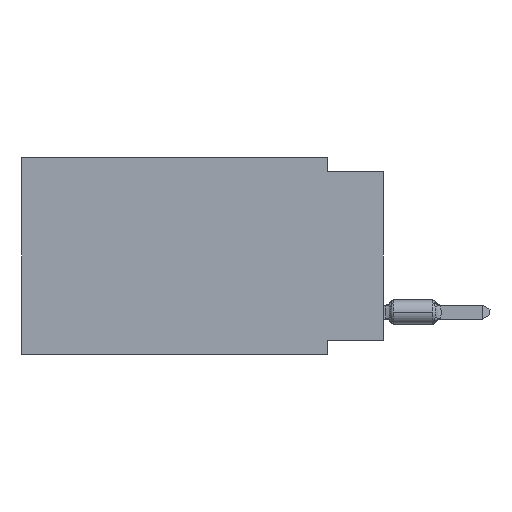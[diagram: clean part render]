
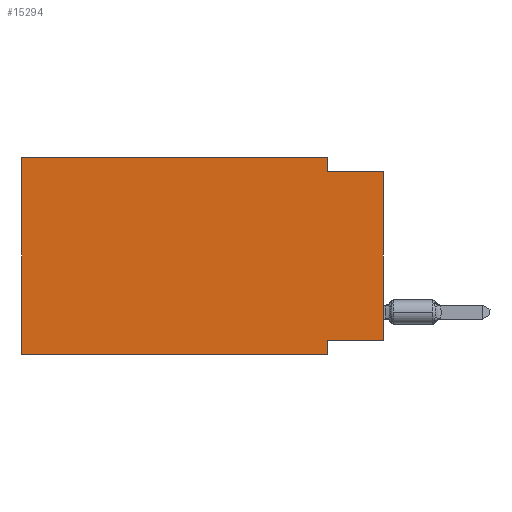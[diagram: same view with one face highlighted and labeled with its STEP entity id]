
A CAD part, left-side view. The second image highlights one B-rep face of the part: STEP entity #15294.
In plain terms, the highlighted planar face has unit normal (-1, 0, 0).
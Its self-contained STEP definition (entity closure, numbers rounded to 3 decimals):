
#206 = VERTEX_POINT ( 'NONE', #7368 ) ;
#236 = CARTESIAN_POINT ( 'NONE',  ( 0., 16.383, 0. ) ) ;
#322 = CARTESIAN_POINT ( 'NONE',  ( 0., 2.54, -8.89 ) ) ;
#358 = VECTOR ( 'NONE', #21157, 1000. ) ;
#823 = VERTEX_POINT ( 'NONE', #1305 ) ;
#853 = VERTEX_POINT ( 'NONE', #322 ) ;
#1194 = LINE ( 'NONE', #21129, #14023 ) ;
#1305 = CARTESIAN_POINT ( 'NONE',  ( 0., 0., -0.635 ) ) ;
#1414 = DIRECTION ( 'NONE',  ( 0., 1., 0. ) ) ;
#1846 = CARTESIAN_POINT ( 'NONE',  ( 0., 0., -0.635 ) ) ;
#2384 = VECTOR ( 'NONE', #6241, 1000. ) ;
#2783 = ORIENTED_EDGE ( 'NONE', *, *, #10857, .T. ) ;
#2955 = CARTESIAN_POINT ( 'NONE',  ( 0., 0., -8.255 ) ) ;
#3058 = ORIENTED_EDGE ( 'NONE', *, *, #7679, .F. ) ;
#3136 = LINE ( 'NONE', #18038, #358 ) ;
#3513 = VECTOR ( 'NONE', #8392, 1000. ) ;
#3583 = ORIENTED_EDGE ( 'NONE', *, *, #16313, .F. ) ;
#3991 = VECTOR ( 'NONE', #20183, 1000. ) ;
#4139 = LINE ( 'NONE', #14010, #7663 ) ;
#4697 = CARTESIAN_POINT ( 'NONE',  ( 0., 16.383, -8.89 ) ) ;
#5078 = EDGE_CURVE ( 'NONE', #13953, #853, #3136, .T. ) ;
#5245 = VERTEX_POINT ( 'NONE', #236 ) ;
#6067 = AXIS2_PLACEMENT_3D ( 'NONE', #10960, #11172, #17395 ) ;
#6167 = VERTEX_POINT ( 'NONE', #20225 ) ;
#6241 = DIRECTION ( 'NONE',  ( 0., 0., 1. ) ) ;
#7368 = CARTESIAN_POINT ( 'NONE',  ( 0., 2.54, -0.635 ) ) ;
#7663 = VECTOR ( 'NONE', #17224, 1000. ) ;
#7679 = EDGE_CURVE ( 'NONE', #206, #823, #18147, .T. ) ;
#7737 = DIRECTION ( 'NONE',  ( 0., -1., 0. ) ) ;
#8152 = EDGE_CURVE ( 'NONE', #19121, #13953, #19838, .T. ) ;
#8179 = CARTESIAN_POINT ( 'NONE',  ( 0., 2.54, 0. ) ) ;
#8392 = DIRECTION ( 'NONE',  ( 0., -1., 0. ) ) ;
#8438 = EDGE_LOOP ( 'NONE', ( #2783, #3058, #14047, #13711, #3583, #16849, #16554, #11705 ) ) ;
#8721 = LINE ( 'NONE', #13652, #3991 ) ;
#9462 = CARTESIAN_POINT ( 'NONE',  ( 0., 0., 0. ) ) ;
#9680 = FACE_OUTER_BOUND ( 'NONE', #8438, .T. ) ;
#9781 = CARTESIAN_POINT ( 'NONE',  ( 0., 0., -8.255 ) ) ;
#10857 = EDGE_CURVE ( 'NONE', #19121, #823, #21034, .T. ) ;
#10960 = CARTESIAN_POINT ( 'NONE',  ( 0., 16.383, 0. ) ) ;
#11172 = DIRECTION ( 'NONE',  ( 1., 0., 0. ) ) ;
#11208 = EDGE_CURVE ( 'NONE', #6167, #853, #19391, .T. ) ;
#11239 = DIRECTION ( 'NONE',  ( 0., -1., 0. ) ) ;
#11705 = ORIENTED_EDGE ( 'NONE', *, *, #8152, .F. ) ;
#12894 = PLANE ( 'NONE',  #6067 ) ;
#13652 = CARTESIAN_POINT ( 'NONE',  ( 0., 16.383, 0. ) ) ;
#13711 = ORIENTED_EDGE ( 'NONE', *, *, #14852, .F. ) ;
#13953 = VERTEX_POINT ( 'NONE', #14702 ) ;
#14010 = CARTESIAN_POINT ( 'NONE',  ( 0., 2.54, 0. ) ) ;
#14023 = VECTOR ( 'NONE', #7737, 1000. ) ;
#14047 = ORIENTED_EDGE ( 'NONE', *, *, #20196, .F. ) ;
#14702 = CARTESIAN_POINT ( 'NONE',  ( 0., 2.54, -8.255 ) ) ;
#14852 = EDGE_CURVE ( 'NONE', #5245, #17685, #1194, .T. ) ;
#15294 = ADVANCED_FACE ( 'NONE', ( #9680 ), #12894, .F. ) ;
#16313 = EDGE_CURVE ( 'NONE', #6167, #5245, #8721, .T. ) ;
#16554 = ORIENTED_EDGE ( 'NONE', *, *, #5078, .F. ) ;
#16849 = ORIENTED_EDGE ( 'NONE', *, *, #11208, .T. ) ;
#17222 = VECTOR ( 'NONE', #1414, 1000. ) ;
#17224 = DIRECTION ( 'NONE',  ( 0., 0., -1. ) ) ;
#17395 = DIRECTION ( 'NONE',  ( 0., 0., -1. ) ) ;
#17413 = VECTOR ( 'NONE', #11239, 1000. ) ;
#17685 = VERTEX_POINT ( 'NONE', #8179 ) ;
#18038 = CARTESIAN_POINT ( 'NONE',  ( 0., 2.54, -8.89 ) ) ;
#18147 = LINE ( 'NONE', #1846, #3513 ) ;
#19121 = VERTEX_POINT ( 'NONE', #2955 ) ;
#19391 = LINE ( 'NONE', #4697, #17413 ) ;
#19838 = LINE ( 'NONE', #9781, #17222 ) ;
#20183 = DIRECTION ( 'NONE',  ( 0., 0., 1. ) ) ;
#20196 = EDGE_CURVE ( 'NONE', #17685, #206, #4139, .T. ) ;
#20225 = CARTESIAN_POINT ( 'NONE',  ( 0., 16.383, -8.89 ) ) ;
#21034 = LINE ( 'NONE', #9462, #2384 ) ;
#21129 = CARTESIAN_POINT ( 'NONE',  ( 0., 16.383, 0. ) ) ;
#21157 = DIRECTION ( 'NONE',  ( 0., 0., -1. ) ) ;
